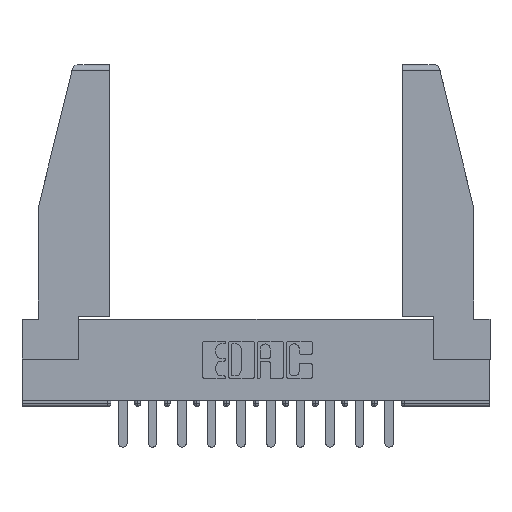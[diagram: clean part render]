
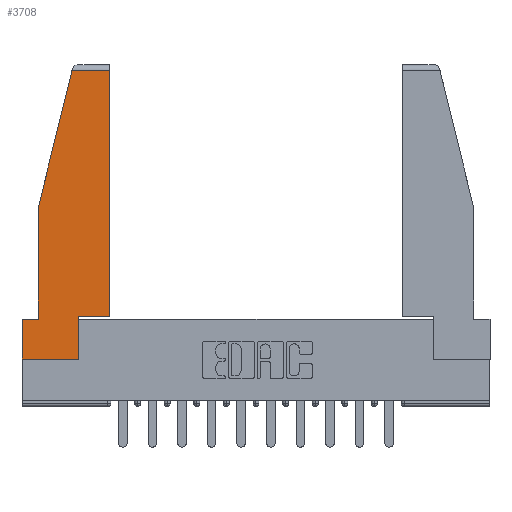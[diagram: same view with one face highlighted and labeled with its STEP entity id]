
A CAD part, top view. The second image highlights one B-rep face of the part: STEP entity #3708.
In plain terms, the highlighted planar face has unit normal (0, 0, 1).
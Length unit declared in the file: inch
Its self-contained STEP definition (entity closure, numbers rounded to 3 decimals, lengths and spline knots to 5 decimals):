
#195 = ORIENTED_EDGE ( 'NONE', *, *, #813, .T. ) ;
#493 = VECTOR ( 'NONE', #7005, 39.37008 ) ;
#813 = EDGE_CURVE ( 'NONE', #15653, #6585, #9683, .T. ) ;
#876 = VERTEX_POINT ( 'NONE', #11600 ) ;
#1472 = CARTESIAN_POINT ( 'NONE',  ( 0.086, 0.8, 0. ) ) ;
#1583 = FACE_OUTER_BOUND ( 'NONE', #4640, .T. ) ;
#1716 = DIRECTION ( 'NONE',  ( 0., -1., 0. ) ) ;
#2370 = DIRECTION ( 'NONE',  ( -1., 0., 0. ) ) ;
#3134 = VERTEX_POINT ( 'NONE', #11016 ) ;
#3377 = ORIENTED_EDGE ( 'NONE', *, *, #9679, .T. ) ;
#3632 = EDGE_CURVE ( 'NONE', #5397, #15653, #14862, .T. ) ;
#3702 = VECTOR ( 'NONE', #13904, 39.37008 ) ;
#3708 = ADVANCED_FACE ( 'NONE', ( #1583 ), #12833, .T. ) ;
#3779 = CARTESIAN_POINT ( 'NONE',  ( 0.086, 0.21, 0. ) ) ;
#3861 = DIRECTION ( 'NONE',  ( 0., 1., 0. ) ) ;
#4370 = VECTOR ( 'NONE', #6570, 39.37008 ) ;
#4527 = CARTESIAN_POINT ( 'NONE',  ( 0., 0., 0. ) ) ;
#4625 = CARTESIAN_POINT ( 'NONE',  ( 0., 0.21, 0. ) ) ;
#4640 = EDGE_LOOP ( 'NONE', ( #13420, #3377, #6046, #6527, #10998, #12848, #8973, #6440, #195 ) ) ;
#4891 = CARTESIAN_POINT ( 'NONE',  ( 0.297, 0., 0. ) ) ;
#5079 = EDGE_CURVE ( 'NONE', #11278, #14608, #15615, .T. ) ;
#5339 = LINE ( 'NONE', #6451, #5832 ) ;
#5397 = VERTEX_POINT ( 'NONE', #12713 ) ;
#5520 = DIRECTION ( 'NONE',  ( 0., 0., 1. ) ) ;
#5601 = CARTESIAN_POINT ( 'NONE',  ( 0., 0., 0. ) ) ;
#5702 = CARTESIAN_POINT ( 'NONE',  ( 0.461, 0.223, 0. ) ) ;
#5789 = LINE ( 'NONE', #11643, #15196 ) ;
#5832 = VECTOR ( 'NONE', #1716, 39.37008 ) ;
#6046 = ORIENTED_EDGE ( 'NONE', *, *, #11052, .T. ) ;
#6440 = ORIENTED_EDGE ( 'NONE', *, *, #3632, .T. ) ;
#6451 = CARTESIAN_POINT ( 'NONE',  ( 0.086, 0.8, 0. ) ) ;
#6527 = ORIENTED_EDGE ( 'NONE', *, *, #12895, .T. ) ;
#6570 = DIRECTION ( 'NONE',  ( 0., 1., 0. ) ) ;
#6585 = VERTEX_POINT ( 'NONE', #8395 ) ;
#6656 = LINE ( 'NONE', #5702, #4370 ) ;
#6664 = LINE ( 'NONE', #11560, #3702 ) ;
#7005 = DIRECTION ( 'NONE',  ( 1., 0., 0. ) ) ;
#7285 = CARTESIAN_POINT ( 'NONE',  ( 0., 0.21, 0. ) ) ;
#7353 = EDGE_CURVE ( 'NONE', #6585, #11228, #6656, .T. ) ;
#7619 = CARTESIAN_POINT ( 'NONE',  ( 0., 1.52, 0. ) ) ;
#8395 = CARTESIAN_POINT ( 'NONE',  ( 0.461, 0.223, 0. ) ) ;
#8495 = DIRECTION ( 'NONE',  ( 1., 0., 0. ) ) ;
#8973 = ORIENTED_EDGE ( 'NONE', *, *, #15256, .T. ) ;
#9109 = DIRECTION ( 'NONE',  ( 1., 0., 0. ) ) ;
#9290 = VECTOR ( 'NONE', #10251, 39.37008 ) ;
#9309 = VERTEX_POINT ( 'NONE', #1472 ) ;
#9679 = EDGE_CURVE ( 'NONE', #11228, #3134, #11239, .T. ) ;
#9683 = LINE ( 'NONE', #14618, #14026 ) ;
#10251 = DIRECTION ( 'NONE',  ( -1., 0., 0. ) ) ;
#10998 = ORIENTED_EDGE ( 'NONE', *, *, #5079, .T. ) ;
#11016 = CARTESIAN_POINT ( 'NONE',  ( 0.2636, 1.52, 0. ) ) ;
#11052 = EDGE_CURVE ( 'NONE', #3134, #9309, #5789, .T. ) ;
#11228 = VERTEX_POINT ( 'NONE', #12053 ) ;
#11239 = LINE ( 'NONE', #7619, #9290 ) ;
#11278 = VERTEX_POINT ( 'NONE', #3779 ) ;
#11560 = CARTESIAN_POINT ( 'NONE',  ( 0., 0.21, 0. ) ) ;
#11600 = CARTESIAN_POINT ( 'NONE',  ( 0., 0., 0. ) ) ;
#11643 = CARTESIAN_POINT ( 'NONE',  ( 0.271, 1.55, 0. ) ) ;
#12053 = CARTESIAN_POINT ( 'NONE',  ( 0.461, 1.52, 0. ) ) ;
#12279 = EDGE_CURVE ( 'NONE', #14608, #876, #6664, .T. ) ;
#12690 = VECTOR ( 'NONE', #3861, 39.37008 ) ;
#12713 = CARTESIAN_POINT ( 'NONE',  ( 0.297, 0., 0. ) ) ;
#12833 = PLANE ( 'NONE',  #15508 ) ;
#12848 = ORIENTED_EDGE ( 'NONE', *, *, #12279, .T. ) ;
#12895 = EDGE_CURVE ( 'NONE', #9309, #11278, #5339, .T. ) ;
#12938 = DIRECTION ( 'NONE',  ( -0.239, -0.971, 0. ) ) ;
#13420 = ORIENTED_EDGE ( 'NONE', *, *, #7353, .T. ) ;
#13904 = DIRECTION ( 'NONE',  ( 0., -1., 0. ) ) ;
#14026 = VECTOR ( 'NONE', #8495, 39.37008 ) ;
#14608 = VERTEX_POINT ( 'NONE', #7285 ) ;
#14618 = CARTESIAN_POINT ( 'NONE',  ( 0.297, 0.223, 0. ) ) ;
#14862 = LINE ( 'NONE', #4891, #12690 ) ;
#14975 = LINE ( 'NONE', #4527, #493 ) ;
#15196 = VECTOR ( 'NONE', #12938, 39.37008 ) ;
#15247 = CARTESIAN_POINT ( 'NONE',  ( 0.297, 0.223, 0. ) ) ;
#15256 = EDGE_CURVE ( 'NONE', #876, #5397, #14975, .T. ) ;
#15471 = VECTOR ( 'NONE', #2370, 39.37008 ) ;
#15508 = AXIS2_PLACEMENT_3D ( 'NONE', #5601, #5520, #9109 ) ;
#15615 = LINE ( 'NONE', #4625, #15471 ) ;
#15653 = VERTEX_POINT ( 'NONE', #15247 ) ;
